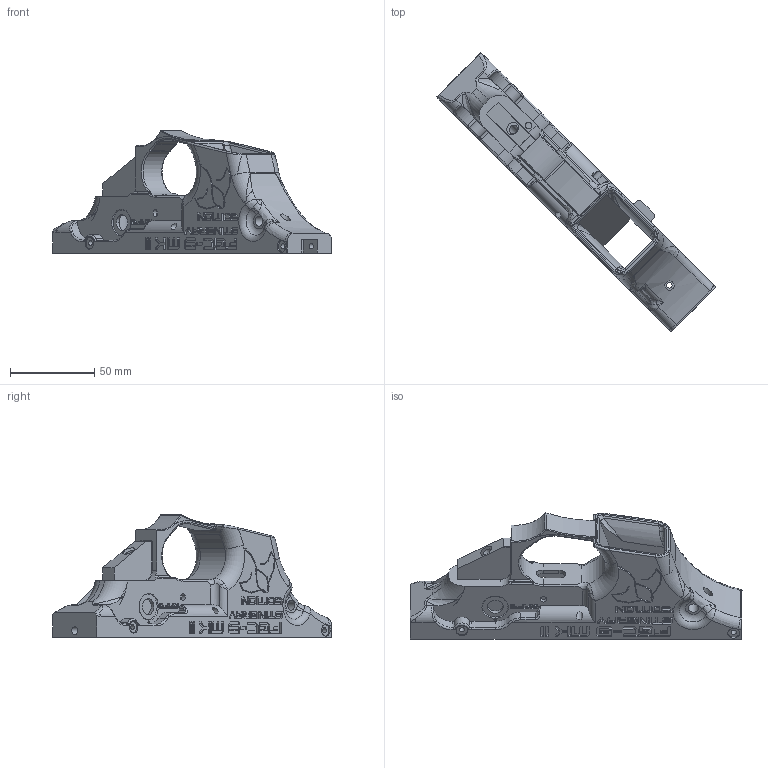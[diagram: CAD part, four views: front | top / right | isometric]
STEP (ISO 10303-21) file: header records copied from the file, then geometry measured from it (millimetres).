
FILE_DESCRIPTION(/* description */ (''),/* implementation_level */ '2;1');
FILE_NAME(/* name */ 'Lower Receiver.step',/* time_stamp */ '2022-05-12T09:39:54-06:00',/* author */ (''),/* organization */ (''),/* preprocessor_version */ 'ST-DEVELOPER v18.1',/* originating_system */ 'Autodesk Translation Framework v10.10.0.1391',/* authorisation */ '');
FILE_SCHEMA (('AUTOMOTIVE_DESIGN { 1 0 10303 214 3 1 1 }'));
Length unit declared in the file: millimetre
Products named in the file (1): Lower Receiver
Bounding box: 165.45 x 165.45 x 72.68 mm (x, y, z)
Volume: 144024.7 mm3; surface area: 51693.7 mm2
Topology: 1 solids, 1 shells, 920 faces, 2540 edges, 1639 vertices
Faces by surface type: plane 598, cylinder 162, bspline 106, torus 47, sphere 5, cone 2
Full cylindrical faces by diameter (mm): 1.5 x1, 3.15 x4, 3.2 x1, 3.75 x1, 4 x4, 4.2 x2, 4.8 x1, 5.2 x1, 5.6 x1, 6 x1, 7.1 x4, 8 x2, 9.5 x2
Entity records: 36776 total; most frequent: CARTESIAN_POINT 13693, ORIENTED_EDGE 5044, DIRECTION 4385, EDGE_CURVE 2522, LINE 1789, VECTOR 1789, VERTEX_POINT 1639, AXIS2_PLACEMENT_3D 1298
